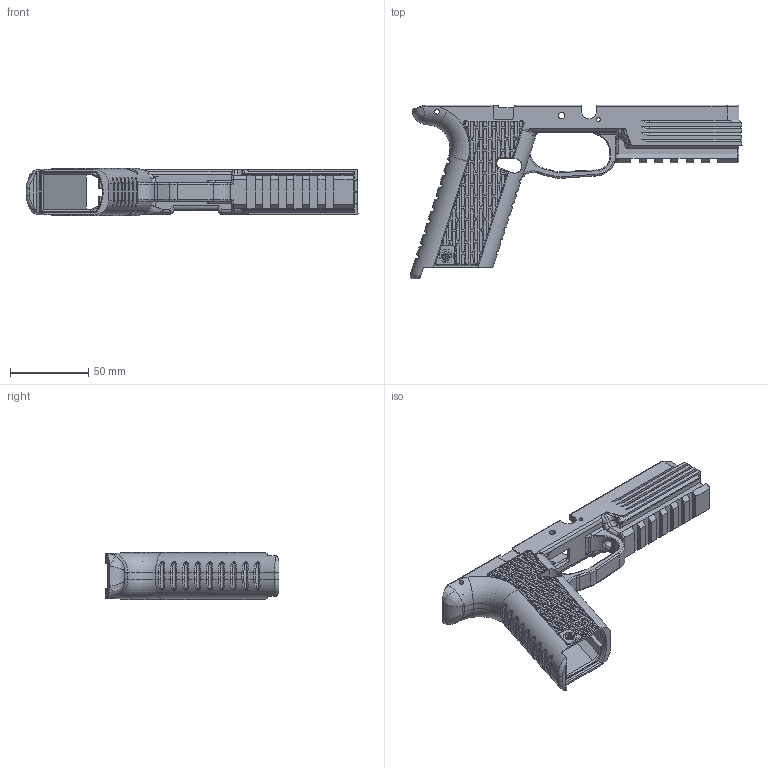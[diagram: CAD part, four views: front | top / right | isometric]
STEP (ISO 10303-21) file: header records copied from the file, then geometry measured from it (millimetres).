
FILE_DESCRIPTION(/* description */ (''),/* implementation_level */ '2;1');
FILE_NAME(/* name */ 'Auto40L.step',/* time_stamp */ '2021-07-12T09:01:11-06:00',/* author */ (''),/* organization */ (''),/* preprocessor_version */ 'ST-DEVELOPER v18.1',/* originating_system */ 'Autodesk Translation Framework v10.9.0.1377',/* authorisation */ '');
FILE_SCHEMA (('AUTOMOTIVE_DESIGN { 1 0 10303 214 3 1 1 }'));
Length unit declared in the file: millimetre
Products named in the file (1): FNS Release
Bounding box: 211.88 x 110.97 x 30.2 mm (x, y, z)
Volume: 120995.7 mm3; surface area: 58093.8 mm2
Topology: 1 solids, 1 shells, 2331 faces, 6400 edges, 4146 vertices
Faces by surface type: bspline 1047, plane 1012, cylinder 212, torus 40, cone 14, sphere 6
Full cylindrical faces by diameter (mm): 2.5 x2, 3 x2, 4.1 x2, 5 x1, 9.75 x1
Entity records: 83618 total; most frequent: CARTESIAN_POINT 34465, ORIENTED_EDGE 12798, DIRECTION 7291, EDGE_CURVE 6399, VERTEX_POINT 4146, LINE 3699, VECTOR 3699, EDGE_LOOP 2431
